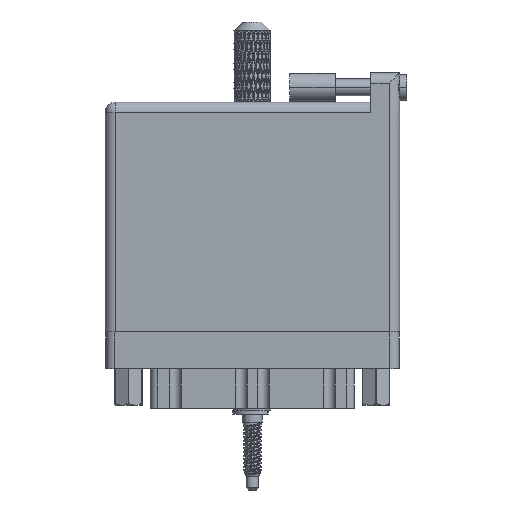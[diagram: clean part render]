
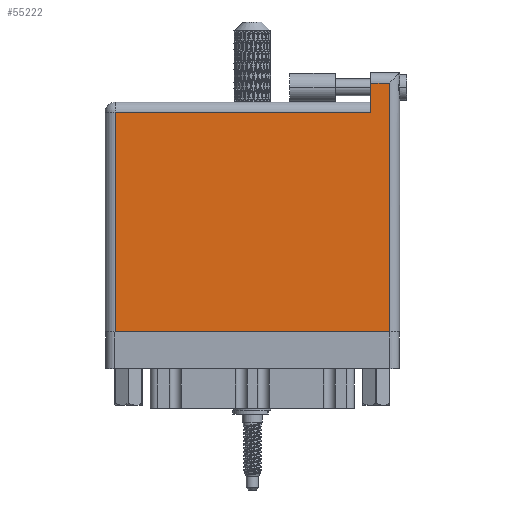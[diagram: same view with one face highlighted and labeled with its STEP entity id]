
A CAD part, front view. The second image highlights one B-rep face of the part: STEP entity #55222.
In plain terms, the highlighted face is planar.
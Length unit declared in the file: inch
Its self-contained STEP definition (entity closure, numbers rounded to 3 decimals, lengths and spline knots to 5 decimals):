
#7451 = VECTOR ( 'NONE', #83951, 39.37008 ) ;
#13881 = VECTOR ( 'NONE', #79802, 39.37008 ) ;
#14160 = ORIENTED_EDGE ( 'NONE', *, *, #61479, .T. ) ;
#14176 = CARTESIAN_POINT ( 'NONE',  ( 1.938, 1.696, 0. ) ) ;
#14202 = CARTESIAN_POINT ( 'NONE',  ( 0., 1.696, 0. ) ) ;
#20730 = CARTESIAN_POINT ( 'NONE',  ( 1.938, 0., 0. ) ) ;
#24779 = EDGE_LOOP ( 'NONE', ( #107266, #109684, #99588, #92555, #14160, #30126 ) ) ;
#25611 = LINE ( 'NONE', #14202, #7451 ) ;
#25670 = CARTESIAN_POINT ( 'NONE',  ( 0., 0., 0. ) ) ;
#25862 = DIRECTION ( 'NONE',  ( 0., -1., 0. ) ) ;
#27217 = VECTOR ( 'NONE', #52463, 39.37008 ) ;
#30126 = ORIENTED_EDGE ( 'NONE', *, *, #104070, .T. ) ;
#30572 = VERTEX_POINT ( 'NONE', #63981 ) ;
#33616 = CARTESIAN_POINT ( 'NONE',  ( 1.811, 1.696, 0. ) ) ;
#36094 = LINE ( 'NONE', #62435, #112662 ) ;
#40999 = FACE_OUTER_BOUND ( 'NONE', #24779, .T. ) ;
#41168 = VERTEX_POINT ( 'NONE', #14176 ) ;
#43364 = LINE ( 'NONE', #25670, #48576 ) ;
#43987 = LINE ( 'NONE', #52009, #86897 ) ;
#46303 = VERTEX_POINT ( 'NONE', #33616 ) ;
#48576 = VECTOR ( 'NONE', #60547, 39.37008 ) ;
#49582 = DIRECTION ( 'NONE',  ( 0., 0., -1. ) ) ;
#52009 = CARTESIAN_POINT ( 'NONE',  ( 1.938, 1.766, 0. ) ) ;
#52463 = DIRECTION ( 'NONE',  ( 0., -1., 0. ) ) ;
#55222 = ADVANCED_FACE ( 'NONE', ( #40999 ), #58740, .F. ) ;
#58740 = PLANE ( 'NONE',  #60353 ) ;
#60353 = AXIS2_PLACEMENT_3D ( 'NONE', #76414, #49582, #75856 ) ;
#60547 = DIRECTION ( 'NONE',  ( 1., 0., 0. ) ) ;
#61479 = EDGE_CURVE ( 'NONE', #89717, #113052, #80942, .T. ) ;
#61968 = EDGE_CURVE ( 'NONE', #72355, #41168, #43987, .T. ) ;
#62435 = CARTESIAN_POINT ( 'NONE',  ( 1.811, 1.766, 0. ) ) ;
#63981 = CARTESIAN_POINT ( 'NONE',  ( 0.07, 0., 0. ) ) ;
#66932 = CARTESIAN_POINT ( 'NONE',  ( 1.811, 1.496, 0. ) ) ;
#68458 = EDGE_CURVE ( 'NONE', #46303, #89717, #36094, .T. ) ;
#72355 = VERTEX_POINT ( 'NONE', #20730 ) ;
#72891 = EDGE_CURVE ( 'NONE', #30572, #72355, #43364, .T. ) ;
#75856 = DIRECTION ( 'NONE',  ( -1., 0., 0. ) ) ;
#76414 = CARTESIAN_POINT ( 'NONE',  ( 0., 1.566, 0. ) ) ;
#79802 = DIRECTION ( 'NONE',  ( -1., 0., 0. ) ) ;
#80942 = LINE ( 'NONE', #106075, #13881 ) ;
#83951 = DIRECTION ( 'NONE',  ( -1., 0., 0. ) ) ;
#86852 = DIRECTION ( 'NONE',  ( 0., 1., 0. ) ) ;
#86897 = VECTOR ( 'NONE', #86852, 39.37008 ) ;
#89717 = VERTEX_POINT ( 'NONE', #66932 ) ;
#90596 = CARTESIAN_POINT ( 'NONE',  ( 0.07, 1.496, 0. ) ) ;
#92555 = ORIENTED_EDGE ( 'NONE', *, *, #68458, .T. ) ;
#95873 = CARTESIAN_POINT ( 'NONE',  ( 0.07, 0., 0. ) ) ;
#96255 = EDGE_CURVE ( 'NONE', #41168, #46303, #25611, .T. ) ;
#99588 = ORIENTED_EDGE ( 'NONE', *, *, #96255, .T. ) ;
#104070 = EDGE_CURVE ( 'NONE', #113052, #30572, #105010, .T. ) ;
#105010 = LINE ( 'NONE', #95873, #27217 ) ;
#106075 = CARTESIAN_POINT ( 'NONE',  ( 0., 1.496, 0. ) ) ;
#107266 = ORIENTED_EDGE ( 'NONE', *, *, #72891, .T. ) ;
#109684 = ORIENTED_EDGE ( 'NONE', *, *, #61968, .T. ) ;
#112662 = VECTOR ( 'NONE', #25862, 39.37008 ) ;
#113052 = VERTEX_POINT ( 'NONE', #90596 ) ;
